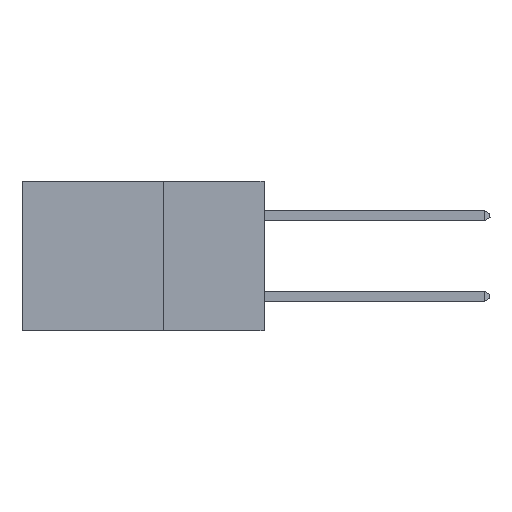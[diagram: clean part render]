
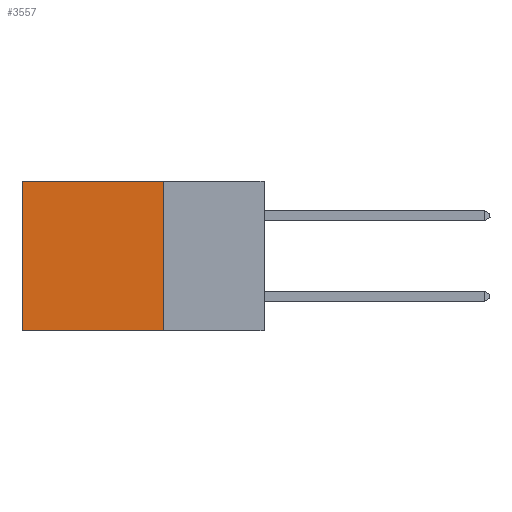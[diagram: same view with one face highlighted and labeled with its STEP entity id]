
A CAD part, left-side view. The second image highlights one B-rep face of the part: STEP entity #3557.
In plain terms, the highlighted planar face has unit normal (-1, 0, 0).
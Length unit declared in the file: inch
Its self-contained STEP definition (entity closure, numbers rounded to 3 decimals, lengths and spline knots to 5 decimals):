
#87 = EDGE_CURVE ( 'NONE', #789, #6283, #8168, .T. ) ;
#186 = CARTESIAN_POINT ( 'NONE',  ( 0.298, 0.25, 0. ) ) ;
#453 = ORIENTED_EDGE ( 'NONE', *, *, #8508, .T. ) ;
#591 = LINE ( 'NONE', #7674, #7401 ) ;
#789 = VERTEX_POINT ( 'NONE', #3088 ) ;
#991 = DIRECTION ( 'NONE',  ( 1., 0., 0. ) ) ;
#1569 = VECTOR ( 'NONE', #4461, 39.37008 ) ;
#1571 = CARTESIAN_POINT ( 'NONE',  ( 0.298, 0.6, 0. ) ) ;
#1898 = VECTOR ( 'NONE', #3851, 39.37008 ) ;
#2346 = CARTESIAN_POINT ( 'NONE',  ( 0.298, 0.25, 0. ) ) ;
#2366 = DIRECTION ( 'NONE',  ( 0., 1., 0. ) ) ;
#2550 = EDGE_LOOP ( 'NONE', ( #453, #8343, #5175, #6816 ) ) ;
#2983 = CARTESIAN_POINT ( 'NONE',  ( 0.298, 0.6, 0. ) ) ;
#3042 = CARTESIAN_POINT ( 'NONE',  ( 0.298, 0.25, 0. ) ) ;
#3088 = CARTESIAN_POINT ( 'NONE',  ( 0.298, 0.25, 0. ) ) ;
#3284 = PLANE ( 'NONE',  #5701 ) ;
#3557 = ADVANCED_FACE ( 'NONE', ( #5751 ), #3284, .F. ) ;
#3851 = DIRECTION ( 'NONE',  ( 0., 1., 0. ) ) ;
#3933 = LINE ( 'NONE', #2346, #1898 ) ;
#4305 = CARTESIAN_POINT ( 'NONE',  ( 0.298, 0.25, -0.37 ) ) ;
#4461 = DIRECTION ( 'NONE',  ( 0., 0., -1. ) ) ;
#5175 = ORIENTED_EDGE ( 'NONE', *, *, #87, .F. ) ;
#5290 = EDGE_CURVE ( 'NONE', #789, #6499, #3933, .T. ) ;
#5618 = LINE ( 'NONE', #2983, #7407 ) ;
#5701 = AXIS2_PLACEMENT_3D ( 'NONE', #186, #991, #7180 ) ;
#5751 = FACE_OUTER_BOUND ( 'NONE', #2550, .T. ) ;
#5753 = EDGE_CURVE ( 'NONE', #6283, #9030, #591, .T. ) ;
#6177 = CARTESIAN_POINT ( 'NONE',  ( 0.298, 0.6, -0.37 ) ) ;
#6283 = VERTEX_POINT ( 'NONE', #4305 ) ;
#6499 = VERTEX_POINT ( 'NONE', #1571 ) ;
#6816 = ORIENTED_EDGE ( 'NONE', *, *, #5290, .T. ) ;
#7180 = DIRECTION ( 'NONE',  ( 0., 0., -1. ) ) ;
#7401 = VECTOR ( 'NONE', #2366, 39.37008 ) ;
#7402 = DIRECTION ( 'NONE',  ( 0., 0., -1. ) ) ;
#7407 = VECTOR ( 'NONE', #7402, 39.37008 ) ;
#7674 = CARTESIAN_POINT ( 'NONE',  ( 0.298, 0.25, -0.37 ) ) ;
#8168 = LINE ( 'NONE', #3042, #1569 ) ;
#8343 = ORIENTED_EDGE ( 'NONE', *, *, #5753, .F. ) ;
#8508 = EDGE_CURVE ( 'NONE', #6499, #9030, #5618, .T. ) ;
#9030 = VERTEX_POINT ( 'NONE', #6177 ) ;
